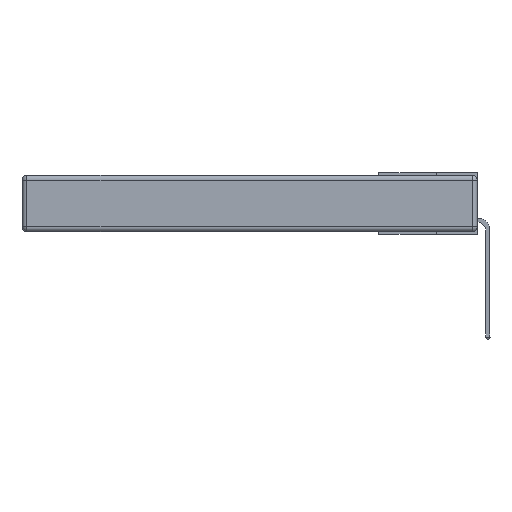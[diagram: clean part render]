
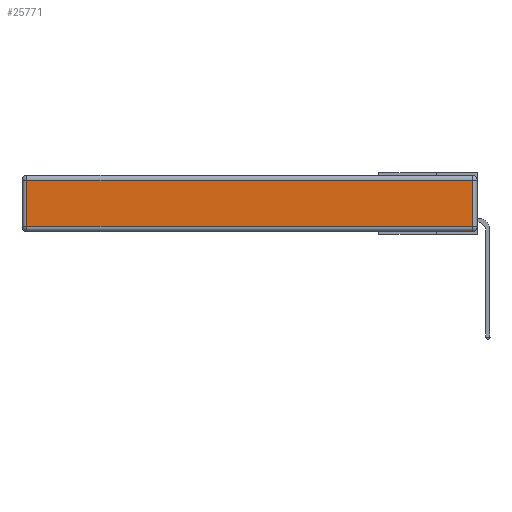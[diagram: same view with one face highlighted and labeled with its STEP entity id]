
A CAD part, left-side view. The second image highlights one B-rep face of the part: STEP entity #25771.
In plain terms, the highlighted planar face has unit normal (-1, 0, 0).
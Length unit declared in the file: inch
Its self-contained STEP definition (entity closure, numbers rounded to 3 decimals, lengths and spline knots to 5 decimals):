
#1649 = VECTOR ( 'NONE', #2705, 39.37008 ) ;
#2203 = EDGE_CURVE ( 'NONE', #6521, #9681, #10083, .T. ) ;
#2705 = DIRECTION ( 'NONE',  ( 0., 1., 0. ) ) ;
#3572 = EDGE_CURVE ( 'NONE', #10072, #6521, #3942, .T. ) ;
#3698 = ORIENTED_EDGE ( 'NONE', *, *, #2203, .T. ) ;
#3850 = PLANE ( 'NONE',  #15296 ) ;
#3942 = LINE ( 'NONE', #9628, #1649 ) ;
#5737 = CARTESIAN_POINT ( 'NONE',  ( 0., 0.03, -0.03 ) ) ;
#6521 = VERTEX_POINT ( 'NONE', #8493 ) ;
#8181 = VECTOR ( 'NONE', #22785, 39.37008 ) ;
#8493 = CARTESIAN_POINT ( 'NONE',  ( 0., 2.72, -0.03 ) ) ;
#9060 = VECTOR ( 'NONE', #10840, 39.37008 ) ;
#9628 = CARTESIAN_POINT ( 'NONE',  ( 0., 2.75, -0.03 ) ) ;
#9681 = VERTEX_POINT ( 'NONE', #20743 ) ;
#10072 = VERTEX_POINT ( 'NONE', #5737 ) ;
#10083 = LINE ( 'NONE', #15490, #8181 ) ;
#10584 = ORIENTED_EDGE ( 'NONE', *, *, #3572, .T. ) ;
#10840 = DIRECTION ( 'NONE',  ( 0., -1., 0. ) ) ;
#11377 = LINE ( 'NONE', #20276, #17106 ) ;
#13738 = EDGE_LOOP ( 'NONE', ( #17161, #26827, #10584, #3698 ) ) ;
#15296 = AXIS2_PLACEMENT_3D ( 'NONE', #20923, #23102, #30403 ) ;
#15490 = CARTESIAN_POINT ( 'NONE',  ( 0., 2.72, -0.343 ) ) ;
#16788 = VERTEX_POINT ( 'NONE', #19007 ) ;
#17106 = VECTOR ( 'NONE', #30162, 39.37008 ) ;
#17161 = ORIENTED_EDGE ( 'NONE', *, *, #21537, .T. ) ;
#19007 = CARTESIAN_POINT ( 'NONE',  ( 0., 0.03, -0.313 ) ) ;
#20004 = FACE_OUTER_BOUND ( 'NONE', #13738, .T. ) ;
#20276 = CARTESIAN_POINT ( 'NONE',  ( 0., 0.03, -0.343 ) ) ;
#20556 = LINE ( 'NONE', #29936, #9060 ) ;
#20743 = CARTESIAN_POINT ( 'NONE',  ( 0., 2.72, -0.313 ) ) ;
#20923 = CARTESIAN_POINT ( 'NONE',  ( 0., 0., -0.343 ) ) ;
#21442 = EDGE_CURVE ( 'NONE', #16788, #10072, #11377, .T. ) ;
#21537 = EDGE_CURVE ( 'NONE', #9681, #16788, #20556, .T. ) ;
#22785 = DIRECTION ( 'NONE',  ( 0., 0., -1. ) ) ;
#23102 = DIRECTION ( 'NONE',  ( -1., 0., 0. ) ) ;
#25771 = ADVANCED_FACE ( 'NONE', ( #20004 ), #3850, .T. ) ;
#26827 = ORIENTED_EDGE ( 'NONE', *, *, #21442, .T. ) ;
#29936 = CARTESIAN_POINT ( 'NONE',  ( 0., 0., -0.313 ) ) ;
#30162 = DIRECTION ( 'NONE',  ( 0., 0., 1. ) ) ;
#30403 = DIRECTION ( 'NONE',  ( 0., 0., 1. ) ) ;
